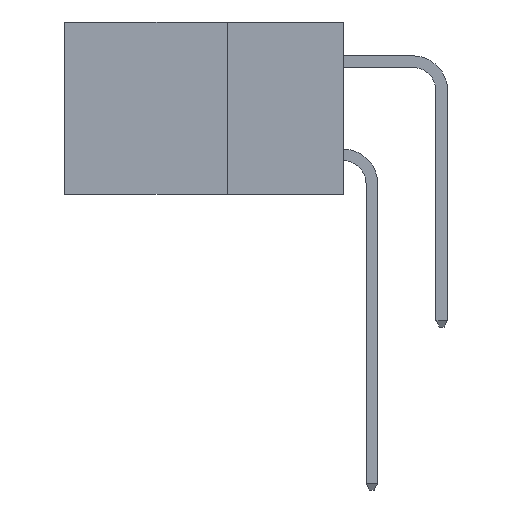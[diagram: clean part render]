
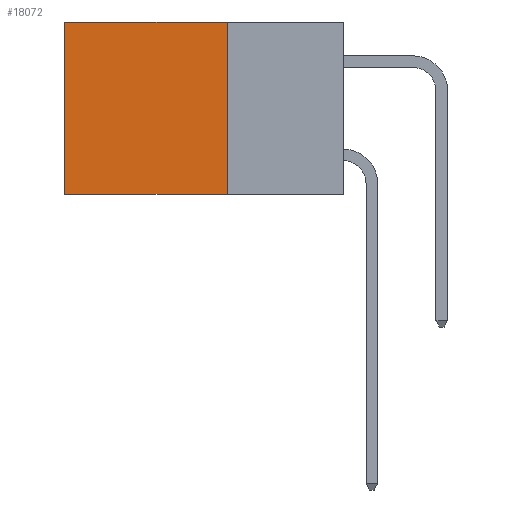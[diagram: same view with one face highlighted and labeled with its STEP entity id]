
A CAD part, left-side view. The second image highlights one B-rep face of the part: STEP entity #18072.
In plain terms, the highlighted planar face has unit normal (-1, 0, 0).
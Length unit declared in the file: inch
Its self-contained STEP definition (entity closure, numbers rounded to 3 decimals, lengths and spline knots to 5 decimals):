
#114 = VERTEX_POINT ( 'NONE', #18782 ) ;
#161 = CARTESIAN_POINT ( 'NONE',  ( 0.2615, 0.25, -0.37 ) ) ;
#239 = DIRECTION ( 'NONE',  ( 1., 0., 0. ) ) ;
#252 = VERTEX_POINT ( 'NONE', #6745 ) ;
#270 = CARTESIAN_POINT ( 'NONE',  ( 0.2615, 0.6, -0.37 ) ) ;
#504 = EDGE_CURVE ( 'NONE', #2973, #252, #10567, .T. ) ;
#1372 = EDGE_CURVE ( 'NONE', #114, #5749, #16324, .T. ) ;
#1629 = EDGE_LOOP ( 'NONE', ( #6334, #13364, #5401, #7588 ) ) ;
#2274 = LINE ( 'NONE', #19835, #2842 ) ;
#2842 = VECTOR ( 'NONE', #9443, 39.37008 ) ;
#2973 = VERTEX_POINT ( 'NONE', #15331 ) ;
#3094 = VECTOR ( 'NONE', #3267, 39.37008 ) ;
#3267 = DIRECTION ( 'NONE',  ( 0., 1., 0. ) ) ;
#5401 = ORIENTED_EDGE ( 'NONE', *, *, #1372, .F. ) ;
#5749 = VERTEX_POINT ( 'NONE', #19921 ) ;
#6144 = DIRECTION ( 'NONE',  ( 0., 0., -1. ) ) ;
#6249 = EDGE_CURVE ( 'NONE', #5749, #252, #2274, .T. ) ;
#6334 = ORIENTED_EDGE ( 'NONE', *, *, #504, .T. ) ;
#6745 = CARTESIAN_POINT ( 'NONE',  ( 0.2615, 0.6, -0.37 ) ) ;
#7499 = PLANE ( 'NONE',  #12226 ) ;
#7588 = ORIENTED_EDGE ( 'NONE', *, *, #14995, .T. ) ;
#9443 = DIRECTION ( 'NONE',  ( 0., 1., 0. ) ) ;
#10567 = LINE ( 'NONE', #270, #15824 ) ;
#11422 = CARTESIAN_POINT ( 'NONE',  ( 0.2615, 0.25, -0.37 ) ) ;
#11618 = VECTOR ( 'NONE', #6144, 39.37008 ) ;
#12226 = AXIS2_PLACEMENT_3D ( 'NONE', #161, #239, #12819 ) ;
#12598 = LINE ( 'NONE', #19077, #3094 ) ;
#12819 = DIRECTION ( 'NONE',  ( 0., 0., -1. ) ) ;
#12851 = DIRECTION ( 'NONE',  ( 0., 0., -1. ) ) ;
#13364 = ORIENTED_EDGE ( 'NONE', *, *, #6249, .F. ) ;
#14995 = EDGE_CURVE ( 'NONE', #114, #2973, #12598, .T. ) ;
#15331 = CARTESIAN_POINT ( 'NONE',  ( 0.2615, 0.6, 0. ) ) ;
#15824 = VECTOR ( 'NONE', #12851, 39.37008 ) ;
#16064 = FACE_OUTER_BOUND ( 'NONE', #1629, .T. ) ;
#16324 = LINE ( 'NONE', #11422, #11618 ) ;
#18072 = ADVANCED_FACE ( 'NONE', ( #16064 ), #7499, .F. ) ;
#18782 = CARTESIAN_POINT ( 'NONE',  ( 0.2615, 0.25, 0. ) ) ;
#19077 = CARTESIAN_POINT ( 'NONE',  ( 0.2615, 0.25, 0. ) ) ;
#19835 = CARTESIAN_POINT ( 'NONE',  ( 0.2615, 0.25, -0.37 ) ) ;
#19921 = CARTESIAN_POINT ( 'NONE',  ( 0.2615, 0.25, -0.37 ) ) ;
